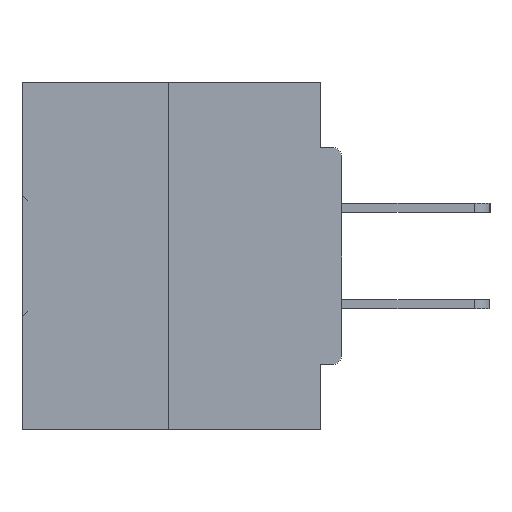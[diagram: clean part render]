
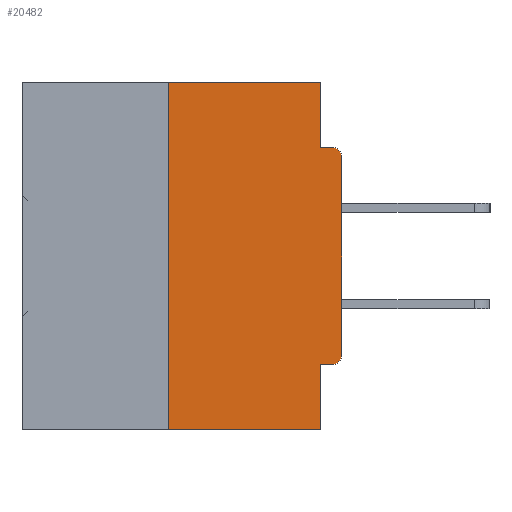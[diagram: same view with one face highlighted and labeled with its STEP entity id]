
A CAD part, left-side view. The second image highlights one B-rep face of the part: STEP entity #20482.
In plain terms, the highlighted planar face has unit normal (-1, 0, 0).
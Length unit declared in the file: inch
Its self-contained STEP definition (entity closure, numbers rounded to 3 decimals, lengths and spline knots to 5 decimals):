
#150 = ORIENTED_EDGE ( 'NONE', *, *, #46391, .T. ) ;
#1039 = VERTEX_POINT ( 'NONE', #6312 ) ;
#1306 = VERTEX_POINT ( 'NONE', #15034 ) ;
#1546 = DIRECTION ( 'NONE',  ( 0., 0., 1. ) ) ;
#2024 = ORIENTED_EDGE ( 'NONE', *, *, #29292, .F. ) ;
#3102 = CARTESIAN_POINT ( 'NONE',  ( 0., 0.031, -0.0935 ) ) ;
#3326 = ORIENTED_EDGE ( 'NONE', *, *, #24292, .T. ) ;
#4649 = DIRECTION ( 'NONE',  ( 0., 0., -1. ) ) ;
#5017 = ORIENTED_EDGE ( 'NONE', *, *, #34375, .F. ) ;
#5161 = ORIENTED_EDGE ( 'NONE', *, *, #41348, .T. ) ;
#5363 = EDGE_CURVE ( 'NONE', #29213, #45218, #17001, .T. ) ;
#5532 = CARTESIAN_POINT ( 'NONE',  ( 0., 0.25, -0.5 ) ) ;
#6312 = CARTESIAN_POINT ( 'NONE',  ( 0., 0.031, 0. ) ) ;
#7018 = DIRECTION ( 'NONE',  ( 0., -1., 0. ) ) ;
#7312 = VECTOR ( 'NONE', #7018, 39.37008 ) ;
#7372 = VECTOR ( 'NONE', #40456, 39.37008 ) ;
#8138 = ORIENTED_EDGE ( 'NONE', *, *, #32227, .F. ) ;
#8592 = DIRECTION ( 'NONE',  ( -1., 0., 0. ) ) ;
#9174 = CARTESIAN_POINT ( 'NONE',  ( 0., 0.031, -0.5 ) ) ;
#11547 = VECTOR ( 'NONE', #28310, 39.37008 ) ;
#11563 = EDGE_CURVE ( 'NONE', #36881, #45218, #40641, .T. ) ;
#14789 = DIRECTION ( 'NONE',  ( 0., 0., -1. ) ) ;
#15034 = CARTESIAN_POINT ( 'NONE',  ( 0., 0.015, -0.0935 ) ) ;
#15171 = VECTOR ( 'NONE', #45631, 39.37008 ) ;
#15880 = CARTESIAN_POINT ( 'NONE',  ( 0., 0.031, 0. ) ) ;
#16538 = AXIS2_PLACEMENT_3D ( 'NONE', #34503, #8592, #26649 ) ;
#17001 = LINE ( 'NONE', #32165, #7312 ) ;
#18203 = LINE ( 'NONE', #40779, #7372 ) ;
#18768 = CARTESIAN_POINT ( 'NONE',  ( 0., 0., -0.3915 ) ) ;
#19071 = DIRECTION ( 'NONE',  ( 0., -1., 0. ) ) ;
#19293 = AXIS2_PLACEMENT_3D ( 'NONE', #25366, #43747, #14789 ) ;
#19932 = VECTOR ( 'NONE', #4649, 39.37008 ) ;
#20482 = ADVANCED_FACE ( 'NONE', ( #40915 ), #29242, .F. ) ;
#20623 = VERTEX_POINT ( 'NONE', #36951 ) ;
#20712 = ORIENTED_EDGE ( 'NONE', *, *, #30543, .F. ) ;
#20969 = CARTESIAN_POINT ( 'NONE',  ( 0., 0.25, 0. ) ) ;
#20972 = DIRECTION ( 'NONE',  ( -1., 0., 0. ) ) ;
#21431 = CIRCLE ( 'NONE', #37017, 0.015 ) ;
#22605 = LINE ( 'NONE', #15880, #15171 ) ;
#22887 = VERTEX_POINT ( 'NONE', #27965 ) ;
#23237 = CARTESIAN_POINT ( 'NONE',  ( 0., 0.015, -0.4065 ) ) ;
#24292 = EDGE_CURVE ( 'NONE', #25996, #22887, #42034, .T. ) ;
#24817 = CARTESIAN_POINT ( 'NONE',  ( 0., 0.015, -0.3915 ) ) ;
#25366 = CARTESIAN_POINT ( 'NONE',  ( 0., 0.46, 0. ) ) ;
#25996 = VERTEX_POINT ( 'NONE', #18768 ) ;
#26649 = DIRECTION ( 'NONE',  ( 0., 0., -1. ) ) ;
#27184 = LINE ( 'NONE', #20969, #43280 ) ;
#27761 = DIRECTION ( 'NONE',  ( 0., 0., -1. ) ) ;
#27965 = CARTESIAN_POINT ( 'NONE',  ( 0., 0., -0.1085 ) ) ;
#28020 = ORIENTED_EDGE ( 'NONE', *, *, #11563, .F. ) ;
#28103 = VERTEX_POINT ( 'NONE', #23237 ) ;
#28310 = DIRECTION ( 'NONE',  ( 0., -1., 0. ) ) ;
#29213 = VERTEX_POINT ( 'NONE', #5532 ) ;
#29242 = PLANE ( 'NONE',  #19293 ) ;
#29292 = EDGE_CURVE ( 'NONE', #29213, #20623, #27184, .T. ) ;
#29497 = VECTOR ( 'NONE', #19071, 39.37008 ) ;
#29918 = CARTESIAN_POINT ( 'NONE',  ( 0., 0.031, -0.5 ) ) ;
#30478 = CARTESIAN_POINT ( 'NONE',  ( 0., 0., 0. ) ) ;
#30543 = EDGE_CURVE ( 'NONE', #32755, #1306, #41974, .T. ) ;
#32133 = EDGE_LOOP ( 'NONE', ( #47280, #2024, #33072, #28020, #8138, #5161, #3326, #150, #20712, #5017 ) ) ;
#32165 = CARTESIAN_POINT ( 'NONE',  ( 0., 0.46, -0.5 ) ) ;
#32227 = EDGE_CURVE ( 'NONE', #28103, #36881, #18203, .T. ) ;
#32229 = VECTOR ( 'NONE', #1546, 39.37008 ) ;
#32405 = LINE ( 'NONE', #33541, #29497 ) ;
#32755 = VERTEX_POINT ( 'NONE', #3102 ) ;
#33072 = ORIENTED_EDGE ( 'NONE', *, *, #5363, .T. ) ;
#33541 = CARTESIAN_POINT ( 'NONE',  ( 0., 0.46, 0. ) ) ;
#34267 = EDGE_CURVE ( 'NONE', #20623, #1039, #32405, .T. ) ;
#34375 = EDGE_CURVE ( 'NONE', #1039, #32755, #22605, .T. ) ;
#34503 = CARTESIAN_POINT ( 'NONE',  ( 0., 0.015, -0.1085 ) ) ;
#36881 = VERTEX_POINT ( 'NONE', #44883 ) ;
#36951 = CARTESIAN_POINT ( 'NONE',  ( 0., 0.25, 0. ) ) ;
#37017 = AXIS2_PLACEMENT_3D ( 'NONE', #24817, #20972, #27761 ) ;
#39409 = CIRCLE ( 'NONE', #16538, 0.015 ) ;
#40456 = DIRECTION ( 'NONE',  ( 0., 1., 0. ) ) ;
#40641 = LINE ( 'NONE', #29918, #19932 ) ;
#40779 = CARTESIAN_POINT ( 'NONE',  ( 0., 0., -0.4065 ) ) ;
#40915 = FACE_OUTER_BOUND ( 'NONE', #32133, .T. ) ;
#41348 = EDGE_CURVE ( 'NONE', #28103, #25996, #21431, .T. ) ;
#41974 = LINE ( 'NONE', #42947, #11547 ) ;
#42034 = LINE ( 'NONE', #30478, #32229 ) ;
#42947 = CARTESIAN_POINT ( 'NONE',  ( 0., 0., -0.0935 ) ) ;
#43280 = VECTOR ( 'NONE', #46287, 39.37008 ) ;
#43747 = DIRECTION ( 'NONE',  ( 1., 0., 0. ) ) ;
#44883 = CARTESIAN_POINT ( 'NONE',  ( 0., 0.031, -0.4065 ) ) ;
#45218 = VERTEX_POINT ( 'NONE', #9174 ) ;
#45631 = DIRECTION ( 'NONE',  ( 0., 0., -1. ) ) ;
#46287 = DIRECTION ( 'NONE',  ( 0., 0., 1. ) ) ;
#46391 = EDGE_CURVE ( 'NONE', #22887, #1306, #39409, .T. ) ;
#47280 = ORIENTED_EDGE ( 'NONE', *, *, #34267, .F. ) ;
